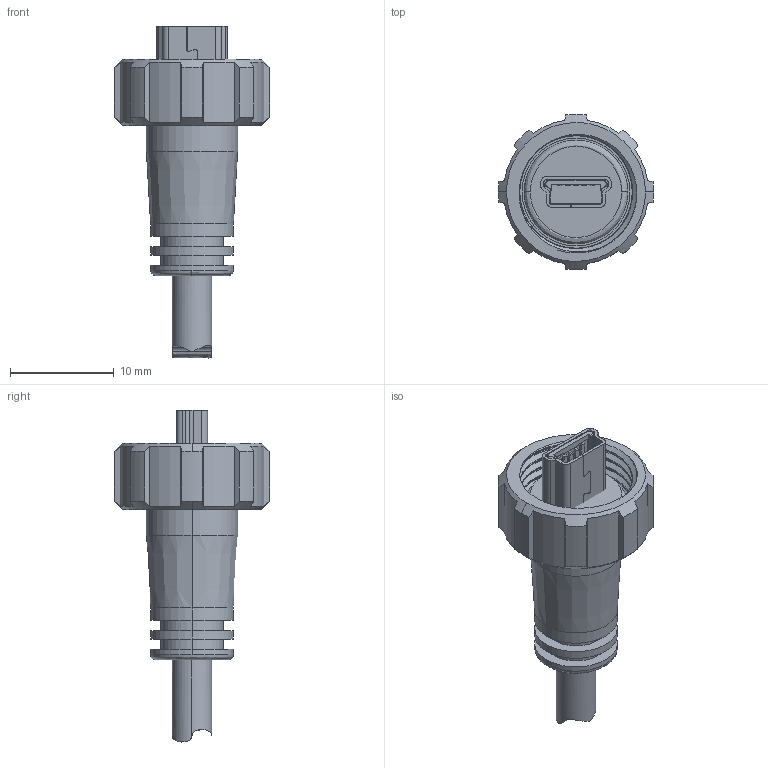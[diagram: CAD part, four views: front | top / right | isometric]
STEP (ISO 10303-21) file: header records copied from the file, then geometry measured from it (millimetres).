
FILE_DESCRIPTION (( 'STEP AP214' ), '1' );
FILE_NAME ('690-W05-260-043.STEP', '2021-04-12T18:31:32', ( '' ), ( '' ), 'SwSTEP 2.0', 'SolidWorks 2020', '' );
FILE_SCHEMA (( 'AUTOMOTIVE_DESIGN' ));
Length unit declared in the file: millimetre
Products named in the file (8): USB ASSY 690-W05-X60-043; USB CONTACTS 690-W05-X60-043; USB SHELL2 690-W05-X60-043; 690-W05-260-043; OVERMOULD 690-W05-X60-043; NUT 690-W05-X60-043; USB SHELL1 690-W05-X60-043; O-RING 690-W05-X60-043
Assembly tree (7 placements, depth 3):
  690-W05-260-043
    USB ASSY 690-W05-X60-043
      USB SHELL1 690-W05-X60-043
      USB SHELL2 690-W05-X60-043
      USB CONTACTS 690-W05-X60-043
    OVERMOULD 690-W05-X60-043
    O-RING 690-W05-X60-043
    NUT 690-W05-X60-043
Bounding box: 15 x 14.99 x 32.03 mm (x, y, z)
Volume: 1732.3 mm3; surface area: 2732.1 mm2
Topology: 9 solids, 9 shells, 568 faces, 1630 edges, 1060 vertices
Faces by surface type: plane 343, cylinder 190, bspline 27, cone 8
Entity records: 23051 total; most frequent: CARTESIAN_POINT 7577, ORIENTED_EDGE 3260, DIRECTION 2871, EDGE_CURVE 1630, VERTEX_POINT 1060, VECTOR 1053, LINE 1053, AXIS2_PLACEMENT_3D 909
